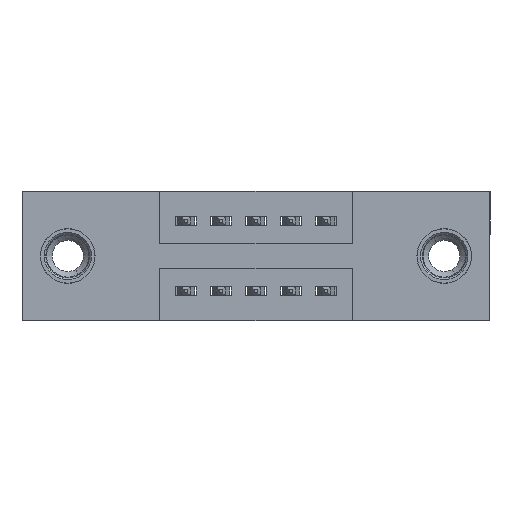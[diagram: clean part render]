
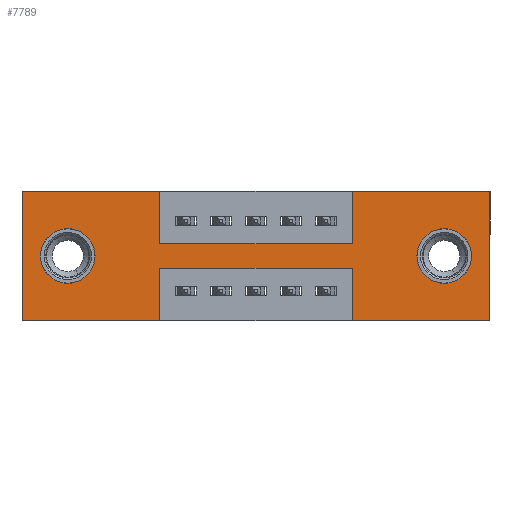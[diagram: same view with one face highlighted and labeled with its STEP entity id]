
A CAD part, front view. The second image highlights one B-rep face of the part: STEP entity #7789.
In plain terms, the highlighted planar face has unit normal (0, -1, 0).
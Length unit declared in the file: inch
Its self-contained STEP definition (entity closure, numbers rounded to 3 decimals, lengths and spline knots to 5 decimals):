
#209 = VERTEX_POINT ( 'NONE', #10691 ) ;
#227 = ORIENTED_EDGE ( 'NONE', *, *, #4089, .T. ) ;
#231 = VERTEX_POINT ( 'NONE', #10756 ) ;
#234 = VERTEX_POINT ( 'NONE', #10892 ) ;
#341 = DIRECTION ( 'NONE',  ( 0., 0., -1. ) ) ;
#359 = VERTEX_POINT ( 'NONE', #6426 ) ;
#530 = CARTESIAN_POINT ( 'NONE',  ( 0.3925, 0., -0.37 ) ) ;
#533 = DIRECTION ( 'NONE',  ( 0., 1., 0. ) ) ;
#573 = CARTESIAN_POINT ( 'NONE',  ( 0.13, 0., -0.263 ) ) ;
#588 = CARTESIAN_POINT ( 'NONE',  ( 1.335, 0., 0. ) ) ;
#624 = AXIS2_PLACEMENT_3D ( 'NONE', #3479, #9288, #4338 ) ;
#634 = DIRECTION ( 'NONE',  ( 0., 0., 1. ) ) ;
#706 = EDGE_LOOP ( 'NONE', ( #227, #5865 ) ) ;
#845 = CARTESIAN_POINT ( 'NONE',  ( 0.3925, 0., -0.15 ) ) ;
#978 = EDGE_CURVE ( 'NONE', #3329, #231, #1362, .T. ) ;
#1035 = LINE ( 'NONE', #8498, #3231 ) ;
#1124 = FACE_BOUND ( 'NONE', #706, .T. ) ;
#1128 = VECTOR ( 'NONE', #4669, 39.37008 ) ;
#1176 = EDGE_CURVE ( 'NONE', #10351, #7125, #1498, .T. ) ;
#1303 = DIRECTION ( 'NONE',  ( 1., 0., 0. ) ) ;
#1311 = VERTEX_POINT ( 'NONE', #2533 ) ;
#1362 = LINE ( 'NONE', #3213, #5852 ) ;
#1376 = DIRECTION ( 'NONE',  ( 0., 1., 0. ) ) ;
#1378 = CARTESIAN_POINT ( 'NONE',  ( 0., 0., 0. ) ) ;
#1428 = VECTOR ( 'NONE', #6271, 39.37008 ) ;
#1453 = CARTESIAN_POINT ( 'NONE',  ( 0.9425, 0., -0.37 ) ) ;
#1473 = EDGE_CURVE ( 'NONE', #4885, #234, #10121, .T. ) ;
#1498 = LINE ( 'NONE', #1378, #5970 ) ;
#1522 = CARTESIAN_POINT ( 'NONE',  ( 1.335, 0., -0.37 ) ) ;
#1584 = DIRECTION ( 'NONE',  ( -1., 0., 0. ) ) ;
#1689 = DIRECTION ( 'NONE',  ( 0., 0., -1. ) ) ;
#1742 = CARTESIAN_POINT ( 'NONE',  ( 1.205, 0., -0.185 ) ) ;
#1846 = ORIENTED_EDGE ( 'NONE', *, *, #6653, .F. ) ;
#1896 = VERTEX_POINT ( 'NONE', #573 ) ;
#1897 = DIRECTION ( 'NONE',  ( 0., 0., 1. ) ) ;
#1962 = EDGE_CURVE ( 'NONE', #359, #1311, #9606, .T. ) ;
#2078 = ORIENTED_EDGE ( 'NONE', *, *, #7351, .F. ) ;
#2335 = AXIS2_PLACEMENT_3D ( 'NONE', #6007, #2482, #8462 ) ;
#2435 = ORIENTED_EDGE ( 'NONE', *, *, #1176, .F. ) ;
#2482 = DIRECTION ( 'NONE',  ( 0., -1., 0. ) ) ;
#2533 = CARTESIAN_POINT ( 'NONE',  ( 0.3925, 0., -0.37 ) ) ;
#2545 = VERTEX_POINT ( 'NONE', #1522 ) ;
#2706 = DIRECTION ( 'NONE',  ( 0., 0., 1. ) ) ;
#2890 = ORIENTED_EDGE ( 'NONE', *, *, #9266, .T. ) ;
#3090 = VERTEX_POINT ( 'NONE', #8854 ) ;
#3131 = VECTOR ( 'NONE', #9272, 39.37008 ) ;
#3162 = ORIENTED_EDGE ( 'NONE', *, *, #978, .F. ) ;
#3187 = VERTEX_POINT ( 'NONE', #9782 ) ;
#3206 = AXIS2_PLACEMENT_3D ( 'NONE', #6679, #1376, #7511 ) ;
#3213 = CARTESIAN_POINT ( 'NONE',  ( 0.9425, 0., -0.37 ) ) ;
#3231 = VECTOR ( 'NONE', #1584, 39.37008 ) ;
#3261 = EDGE_CURVE ( 'NONE', #1896, #5706, #7926, .T. ) ;
#3329 = VERTEX_POINT ( 'NONE', #1453 ) ;
#3411 = LINE ( 'NONE', #7832, #10008 ) ;
#3455 = CARTESIAN_POINT ( 'NONE',  ( 0., 0., 0. ) ) ;
#3479 = CARTESIAN_POINT ( 'NONE',  ( 0.13, 0., -0.185 ) ) ;
#3596 = FACE_OUTER_BOUND ( 'NONE', #9052, .T. ) ;
#3875 = LINE ( 'NONE', #8705, #1428 ) ;
#4033 = ORIENTED_EDGE ( 'NONE', *, *, #8543, .F. ) ;
#4089 = EDGE_CURVE ( 'NONE', #5706, #1896, #6760, .T. ) ;
#4204 = EDGE_CURVE ( 'NONE', #4559, #10351, #3411, .T. ) ;
#4338 = DIRECTION ( 'NONE',  ( 0., 0., 1. ) ) ;
#4559 = VERTEX_POINT ( 'NONE', #10607 ) ;
#4669 = DIRECTION ( 'NONE',  ( -1., 0., 0. ) ) ;
#4744 = VECTOR ( 'NONE', #634, 39.37008 ) ;
#4884 = CARTESIAN_POINT ( 'NONE',  ( 1.335, 0., 0. ) ) ;
#4885 = VERTEX_POINT ( 'NONE', #10173 ) ;
#4923 = LINE ( 'NONE', #10142, #9023 ) ;
#5045 = ORIENTED_EDGE ( 'NONE', *, *, #1473, .T. ) ;
#5237 = VECTOR ( 'NONE', #9790, 39.37008 ) ;
#5379 = DIRECTION ( 'NONE',  ( 0., 1., 0. ) ) ;
#5482 = EDGE_CURVE ( 'NONE', #7755, #3090, #9115, .T. ) ;
#5576 = VECTOR ( 'NONE', #341, 39.37008 ) ;
#5706 = VERTEX_POINT ( 'NONE', #6376 ) ;
#5852 = VECTOR ( 'NONE', #1897, 39.37008 ) ;
#5865 = ORIENTED_EDGE ( 'NONE', *, *, #3261, .T. ) ;
#5875 = EDGE_CURVE ( 'NONE', #231, #359, #1035, .T. ) ;
#5907 = FACE_BOUND ( 'NONE', #8055, .T. ) ;
#5909 = LINE ( 'NONE', #7179, #1128 ) ;
#5934 = CARTESIAN_POINT ( 'NONE',  ( 1.205, 0., -0.185 ) ) ;
#5954 = ORIENTED_EDGE ( 'NONE', *, *, #4204, .F. ) ;
#5970 = VECTOR ( 'NONE', #1303, 39.37008 ) ;
#6007 = CARTESIAN_POINT ( 'NONE',  ( 0., 0., -0.37 ) ) ;
#6271 = DIRECTION ( 'NONE',  ( 0., 0., -1. ) ) ;
#6325 = ORIENTED_EDGE ( 'NONE', *, *, #1962, .F. ) ;
#6376 = CARTESIAN_POINT ( 'NONE',  ( 0.13, 0., -0.107 ) ) ;
#6426 = CARTESIAN_POINT ( 'NONE',  ( 0.3925, 0., -0.22 ) ) ;
#6527 = CARTESIAN_POINT ( 'NONE',  ( 0.9425, 0., 0. ) ) ;
#6653 = EDGE_CURVE ( 'NONE', #3187, #4559, #10586, .T. ) ;
#6679 = CARTESIAN_POINT ( 'NONE',  ( 0.13, 0., -0.185 ) ) ;
#6691 = ORIENTED_EDGE ( 'NONE', *, *, #5482, .F. ) ;
#6760 = CIRCLE ( 'NONE', #624, 0.078 ) ;
#6766 = DIRECTION ( 'NONE',  ( 0., 0., -1. ) ) ;
#7125 = VERTEX_POINT ( 'NONE', #588 ) ;
#7179 = CARTESIAN_POINT ( 'NONE',  ( 0., 0., -0.37 ) ) ;
#7351 = EDGE_CURVE ( 'NONE', #209, #3187, #3875, .T. ) ;
#7403 = ORIENTED_EDGE ( 'NONE', *, *, #5875, .F. ) ;
#7511 = DIRECTION ( 'NONE',  ( 0., 0., 1. ) ) ;
#7637 = AXIS2_PLACEMENT_3D ( 'NONE', #5934, #533, #6766 ) ;
#7656 = LINE ( 'NONE', #8484, #3131 ) ;
#7657 = PLANE ( 'NONE',  #2335 ) ;
#7755 = VERTEX_POINT ( 'NONE', #8432 ) ;
#7789 = ADVANCED_FACE ( 'NONE', ( #5907, #1124, #3596 ), #7657, .T. ) ;
#7832 = CARTESIAN_POINT ( 'NONE',  ( 0.9425, 0., 0. ) ) ;
#7851 = DIRECTION ( 'NONE',  ( 1., 0., 0. ) ) ;
#7880 = AXIS2_PLACEMENT_3D ( 'NONE', #1742, #5379, #1689 ) ;
#7926 = CIRCLE ( 'NONE', #3206, 0.078 ) ;
#8055 = EDGE_LOOP ( 'NONE', ( #5045, #2890 ) ) ;
#8096 = EDGE_CURVE ( 'NONE', #7125, #2545, #10052, .T. ) ;
#8394 = ORIENTED_EDGE ( 'NONE', *, *, #10071, .F. ) ;
#8432 = CARTESIAN_POINT ( 'NONE',  ( 0., 0., -0.37 ) ) ;
#8462 = DIRECTION ( 'NONE',  ( 0., 0., -1. ) ) ;
#8484 = CARTESIAN_POINT ( 'NONE',  ( 0., 0., -0.37 ) ) ;
#8498 = CARTESIAN_POINT ( 'NONE',  ( 0.3925, 0., -0.22 ) ) ;
#8543 = EDGE_CURVE ( 'NONE', #2545, #3329, #5909, .T. ) ;
#8705 = CARTESIAN_POINT ( 'NONE',  ( 0.3925, 0., 0. ) ) ;
#8854 = CARTESIAN_POINT ( 'NONE',  ( 0., 0., 0. ) ) ;
#9023 = VECTOR ( 'NONE', #9339, 39.37008 ) ;
#9052 = EDGE_LOOP ( 'NONE', ( #6325, #7403, #3162, #4033, #9778, #2435, #5954, #1846, #2078, #8394, #6691, #9166 ) ) ;
#9115 = LINE ( 'NONE', #3455, #4744 ) ;
#9166 = ORIENTED_EDGE ( 'NONE', *, *, #9992, .F. ) ;
#9266 = EDGE_CURVE ( 'NONE', #234, #4885, #9286, .T. ) ;
#9272 = DIRECTION ( 'NONE',  ( -1., 0., 0. ) ) ;
#9286 = CIRCLE ( 'NONE', #7637, 0.078 ) ;
#9288 = DIRECTION ( 'NONE',  ( 0., 1., 0. ) ) ;
#9339 = DIRECTION ( 'NONE',  ( 1., 0., 0. ) ) ;
#9606 = LINE ( 'NONE', #530, #5576 ) ;
#9778 = ORIENTED_EDGE ( 'NONE', *, *, #8096, .F. ) ;
#9782 = CARTESIAN_POINT ( 'NONE',  ( 0.3925, 0., -0.15 ) ) ;
#9790 = DIRECTION ( 'NONE',  ( 0., 0., -1. ) ) ;
#9992 = EDGE_CURVE ( 'NONE', #1311, #7755, #7656, .T. ) ;
#10008 = VECTOR ( 'NONE', #2706, 39.37008 ) ;
#10052 = LINE ( 'NONE', #4884, #5237 ) ;
#10071 = EDGE_CURVE ( 'NONE', #3090, #209, #4923, .T. ) ;
#10121 = CIRCLE ( 'NONE', #7880, 0.078 ) ;
#10142 = CARTESIAN_POINT ( 'NONE',  ( 0., 0., 0. ) ) ;
#10173 = CARTESIAN_POINT ( 'NONE',  ( 1.205, 0., -0.107 ) ) ;
#10333 = VECTOR ( 'NONE', #7851, 39.37008 ) ;
#10351 = VERTEX_POINT ( 'NONE', #6527 ) ;
#10586 = LINE ( 'NONE', #845, #10333 ) ;
#10607 = CARTESIAN_POINT ( 'NONE',  ( 0.9425, 0., -0.15 ) ) ;
#10691 = CARTESIAN_POINT ( 'NONE',  ( 0.3925, 0., 0. ) ) ;
#10756 = CARTESIAN_POINT ( 'NONE',  ( 0.9425, 0., -0.22 ) ) ;
#10892 = CARTESIAN_POINT ( 'NONE',  ( 1.205, 0., -0.263 ) ) ;
